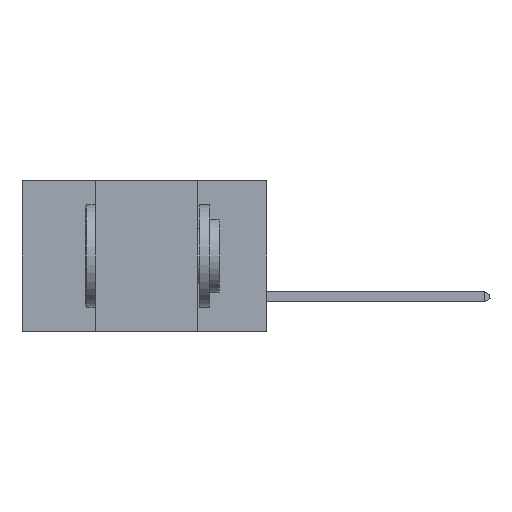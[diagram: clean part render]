
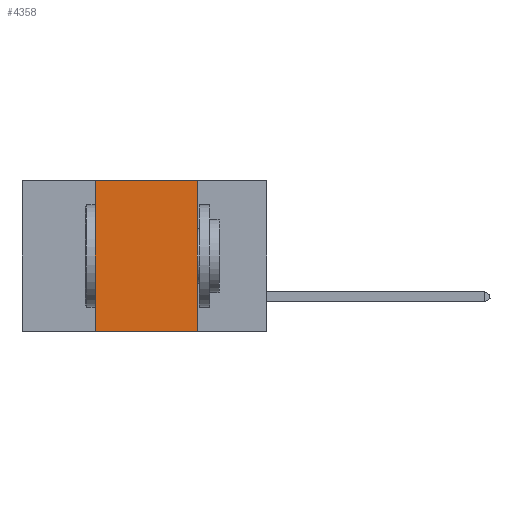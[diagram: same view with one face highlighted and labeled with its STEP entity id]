
A CAD part, left-side view. The second image highlights one B-rep face of the part: STEP entity #4358.
In plain terms, the highlighted planar face has unit normal (-1, 0, 0).
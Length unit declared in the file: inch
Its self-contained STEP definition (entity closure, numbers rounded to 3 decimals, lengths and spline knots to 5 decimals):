
#114 = AXIS2_PLACEMENT_3D ( 'NONE', #37364, #40670, #5331 ) ;
#1281 = LINE ( 'NONE', #14583, #24607 ) ;
#1450 = DIRECTION ( 'NONE',  ( 0., 0., -1. ) ) ;
#4178 = LINE ( 'NONE', #35175, #31431 ) ;
#4358 = ADVANCED_FACE ( 'NONE', ( #13372 ), #5468, .F. ) ;
#5331 = DIRECTION ( 'NONE',  ( 0., 0., -1. ) ) ;
#5468 = PLANE ( 'NONE',  #114 ) ;
#7161 = VECTOR ( 'NONE', #1450, 39.37008 ) ;
#7397 = CARTESIAN_POINT ( 'NONE',  ( 0., 0.17, 0. ) ) ;
#8615 = EDGE_CURVE ( 'NONE', #36283, #8714, #1281, .T. ) ;
#8714 = VERTEX_POINT ( 'NONE', #20562 ) ;
#10987 = DIRECTION ( 'NONE',  ( 0., -1., 0. ) ) ;
#11156 = CARTESIAN_POINT ( 'NONE',  ( 0., 0.17, 0. ) ) ;
#13372 = FACE_OUTER_BOUND ( 'NONE', #35068, .T. ) ;
#14516 = EDGE_CURVE ( 'NONE', #24434, #8714, #28967, .T. ) ;
#14583 = CARTESIAN_POINT ( 'NONE',  ( 0., 0.6, -0.37 ) ) ;
#15719 = CARTESIAN_POINT ( 'NONE',  ( 0., 0.42, 0. ) ) ;
#16181 = ORIENTED_EDGE ( 'NONE', *, *, #14516, .F. ) ;
#18246 = ORIENTED_EDGE ( 'NONE', *, *, #34379, .F. ) ;
#18979 = DIRECTION ( 'NONE',  ( 0., -1., 0. ) ) ;
#20055 = VERTEX_POINT ( 'NONE', #15719 ) ;
#20562 = CARTESIAN_POINT ( 'NONE',  ( 0., 0.17, -0.37 ) ) ;
#21641 = ORIENTED_EDGE ( 'NONE', *, *, #8615, .T. ) ;
#23496 = VECTOR ( 'NONE', #35306, 39.37008 ) ;
#24434 = VERTEX_POINT ( 'NONE', #7397 ) ;
#24607 = VECTOR ( 'NONE', #10987, 39.37008 ) ;
#25473 = CARTESIAN_POINT ( 'NONE',  ( 0., 0.42, 0. ) ) ;
#27868 = CARTESIAN_POINT ( 'NONE',  ( 0., 0.42, -0.37 ) ) ;
#28967 = LINE ( 'NONE', #11156, #7161 ) ;
#29300 = EDGE_CURVE ( 'NONE', #20055, #24434, #4178, .T. ) ;
#29419 = LINE ( 'NONE', #25473, #23496 ) ;
#31429 = ORIENTED_EDGE ( 'NONE', *, *, #29300, .F. ) ;
#31431 = VECTOR ( 'NONE', #18979, 39.37008 ) ;
#34379 = EDGE_CURVE ( 'NONE', #36283, #20055, #29419, .T. ) ;
#35068 = EDGE_LOOP ( 'NONE', ( #16181, #31429, #18246, #21641 ) ) ;
#35175 = CARTESIAN_POINT ( 'NONE',  ( 0., 0.6, 0. ) ) ;
#35306 = DIRECTION ( 'NONE',  ( 0., 0., 1. ) ) ;
#36283 = VERTEX_POINT ( 'NONE', #27868 ) ;
#37364 = CARTESIAN_POINT ( 'NONE',  ( 0., 0.6, 0. ) ) ;
#40670 = DIRECTION ( 'NONE',  ( 1., 0., 0. ) ) ;
